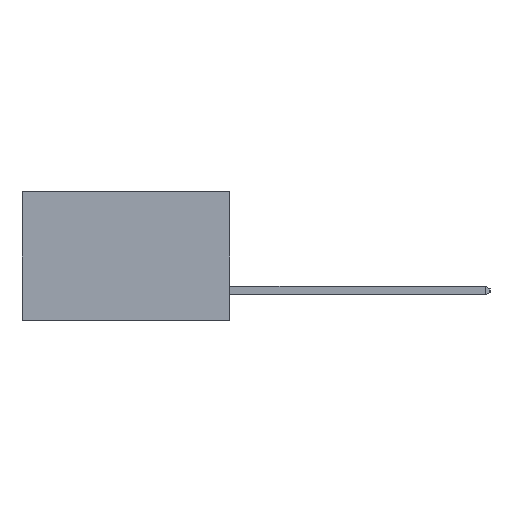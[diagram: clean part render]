
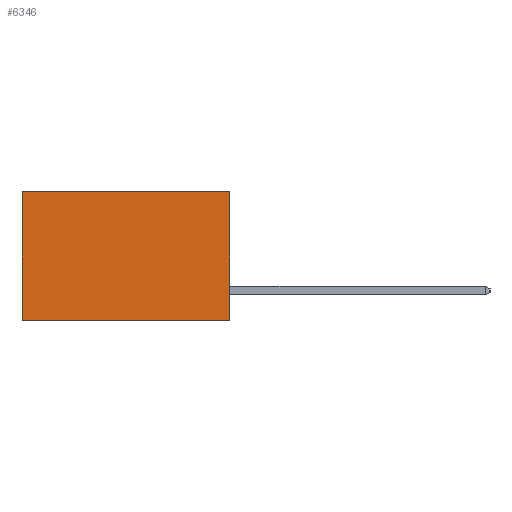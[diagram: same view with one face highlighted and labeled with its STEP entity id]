
A CAD part, left-side view. The second image highlights one B-rep face of the part: STEP entity #6346.
In plain terms, the highlighted planar face has unit normal (-1, 0, 0).
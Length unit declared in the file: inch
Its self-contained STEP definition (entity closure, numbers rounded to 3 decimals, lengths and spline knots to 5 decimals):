
#1214 = EDGE_CURVE ( 'NONE', #16867, #14604, #6985, .T. ) ;
#1220 = LINE ( 'NONE', #16440, #14988 ) ;
#1414 = DIRECTION ( 'NONE',  ( 0., 0., -1. ) ) ;
#1592 = CARTESIAN_POINT ( 'NONE',  ( 0.2615, 0., -0.37 ) ) ;
#1686 = VERTEX_POINT ( 'NONE', #16814 ) ;
#3133 = CARTESIAN_POINT ( 'NONE',  ( 0.2615, 0., 0. ) ) ;
#3591 = LINE ( 'NONE', #11565, #16981 ) ;
#4152 = AXIS2_PLACEMENT_3D ( 'NONE', #16267, #16229, #16191 ) ;
#4227 = DIRECTION ( 'NONE',  ( 0., 1., 0. ) ) ;
#4870 = FACE_OUTER_BOUND ( 'NONE', #13170, .T. ) ;
#6346 = ADVANCED_FACE ( 'NONE', ( #4870 ), #16301, .F. ) ;
#6985 = LINE ( 'NONE', #3133, #10122 ) ;
#7805 = ORIENTED_EDGE ( 'NONE', *, *, #1214, .T. ) ;
#7896 = EDGE_CURVE ( 'NONE', #16867, #16806, #15720, .T. ) ;
#7963 = EDGE_CURVE ( 'NONE', #16806, #1686, #1220, .T. ) ;
#8424 = EDGE_CURVE ( 'NONE', #14604, #1686, #3591, .T. ) ;
#8804 = VECTOR ( 'NONE', #1414, 39.37008 ) ;
#9034 = CARTESIAN_POINT ( 'NONE',  ( 0.2615, 0., 0. ) ) ;
#10122 = VECTOR ( 'NONE', #4227, 39.37008 ) ;
#10266 = ORIENTED_EDGE ( 'NONE', *, *, #7963, .F. ) ;
#10495 = ORIENTED_EDGE ( 'NONE', *, *, #8424, .T. ) ;
#11529 = DIRECTION ( 'NONE',  ( 0., 0., -1. ) ) ;
#11565 = CARTESIAN_POINT ( 'NONE',  ( 0.2615, 0.6, -0.37 ) ) ;
#13170 = EDGE_LOOP ( 'NONE', ( #10495, #10266, #16894, #7805 ) ) ;
#14604 = VERTEX_POINT ( 'NONE', #16431 ) ;
#14988 = VECTOR ( 'NONE', #16933, 39.37008 ) ;
#15444 = CARTESIAN_POINT ( 'NONE',  ( 0.2615, 0., -0.37 ) ) ;
#15720 = LINE ( 'NONE', #1592, #8804 ) ;
#16191 = DIRECTION ( 'NONE',  ( 0., 0., -1. ) ) ;
#16229 = DIRECTION ( 'NONE',  ( 1., 0., 0. ) ) ;
#16267 = CARTESIAN_POINT ( 'NONE',  ( 0.2615, 0., -0.37 ) ) ;
#16301 = PLANE ( 'NONE',  #4152 ) ;
#16431 = CARTESIAN_POINT ( 'NONE',  ( 0.2615, 0.6, 0. ) ) ;
#16440 = CARTESIAN_POINT ( 'NONE',  ( 0.2615, 0., -0.37 ) ) ;
#16806 = VERTEX_POINT ( 'NONE', #15444 ) ;
#16814 = CARTESIAN_POINT ( 'NONE',  ( 0.2615, 0.6, -0.37 ) ) ;
#16867 = VERTEX_POINT ( 'NONE', #9034 ) ;
#16894 = ORIENTED_EDGE ( 'NONE', *, *, #7896, .F. ) ;
#16933 = DIRECTION ( 'NONE',  ( 0., 1., 0. ) ) ;
#16981 = VECTOR ( 'NONE', #11529, 39.37008 ) ;
